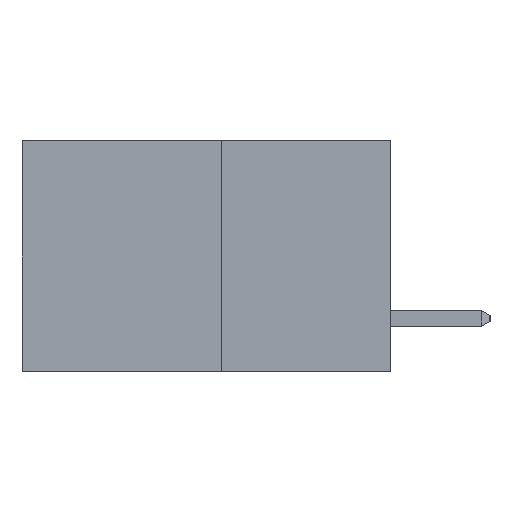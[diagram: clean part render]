
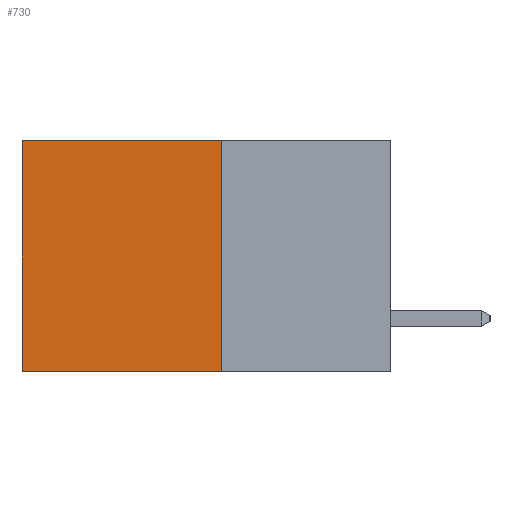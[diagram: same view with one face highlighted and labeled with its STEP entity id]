
A CAD part, left-side view. The second image highlights one B-rep face of the part: STEP entity #730.
In plain terms, the highlighted planar face has unit normal (-1, 0, 0).
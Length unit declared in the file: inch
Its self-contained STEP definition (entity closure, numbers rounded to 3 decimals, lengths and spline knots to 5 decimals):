
#94 = VECTOR ( 'NONE', #2295, 39.37008 ) ;
#142 = EDGE_CURVE ( 'NONE', #12200, #9027, #11539, .T. ) ;
#613 = DIRECTION ( 'NONE',  ( 0., 0., -1. ) ) ;
#663 = DIRECTION ( 'NONE',  ( 1., 0., 0. ) ) ;
#730 = ADVANCED_FACE ( 'NONE', ( #7603 ), #10502, .F. ) ;
#776 = LINE ( 'NONE', #9963, #9222 ) ;
#1023 = CARTESIAN_POINT ( 'NONE',  ( 0.277, 0.59, 0. ) ) ;
#1190 = VERTEX_POINT ( 'NONE', #5155 ) ;
#1852 = LINE ( 'NONE', #11809, #10148 ) ;
#1958 = EDGE_CURVE ( 'NONE', #7594, #9027, #5270, .T. ) ;
#2192 = CARTESIAN_POINT ( 'NONE',  ( 0.277, 0.59, -0.37 ) ) ;
#2295 = DIRECTION ( 'NONE',  ( 0., 0., -1. ) ) ;
#2637 = VECTOR ( 'NONE', #13346, 39.37008 ) ;
#3785 = ORIENTED_EDGE ( 'NONE', *, *, #4339, .T. ) ;
#4252 = EDGE_CURVE ( 'NONE', #1190, #7594, #1852, .T. ) ;
#4339 = EDGE_CURVE ( 'NONE', #1190, #12200, #776, .T. ) ;
#5155 = CARTESIAN_POINT ( 'NONE',  ( 0.277, 0.27, 0. ) ) ;
#5270 = LINE ( 'NONE', #13356, #2637 ) ;
#5503 = AXIS2_PLACEMENT_3D ( 'NONE', #10467, #663, #613 ) ;
#5666 = ORIENTED_EDGE ( 'NONE', *, *, #142, .T. ) ;
#6877 = DIRECTION ( 'NONE',  ( 0., 1., 0. ) ) ;
#7143 = EDGE_LOOP ( 'NONE', ( #5666, #12303, #9366, #3785 ) ) ;
#7594 = VERTEX_POINT ( 'NONE', #13553 ) ;
#7603 = FACE_OUTER_BOUND ( 'NONE', #7143, .T. ) ;
#9027 = VERTEX_POINT ( 'NONE', #9057 ) ;
#9057 = CARTESIAN_POINT ( 'NONE',  ( 0.277, 0.59, -0.37 ) ) ;
#9222 = VECTOR ( 'NONE', #6877, 39.37008 ) ;
#9366 = ORIENTED_EDGE ( 'NONE', *, *, #4252, .F. ) ;
#9963 = CARTESIAN_POINT ( 'NONE',  ( 0.277, 0.27, 0. ) ) ;
#10148 = VECTOR ( 'NONE', #12789, 39.37008 ) ;
#10467 = CARTESIAN_POINT ( 'NONE',  ( 0.277, 0.27, -0.37 ) ) ;
#10502 = PLANE ( 'NONE',  #5503 ) ;
#11539 = LINE ( 'NONE', #2192, #94 ) ;
#11809 = CARTESIAN_POINT ( 'NONE',  ( 0.277, 0.27, -0.37 ) ) ;
#12200 = VERTEX_POINT ( 'NONE', #1023 ) ;
#12303 = ORIENTED_EDGE ( 'NONE', *, *, #1958, .F. ) ;
#12789 = DIRECTION ( 'NONE',  ( 0., 0., -1. ) ) ;
#13346 = DIRECTION ( 'NONE',  ( 0., 1., 0. ) ) ;
#13356 = CARTESIAN_POINT ( 'NONE',  ( 0.277, 0.27, -0.37 ) ) ;
#13553 = CARTESIAN_POINT ( 'NONE',  ( 0.277, 0.27, -0.37 ) ) ;
